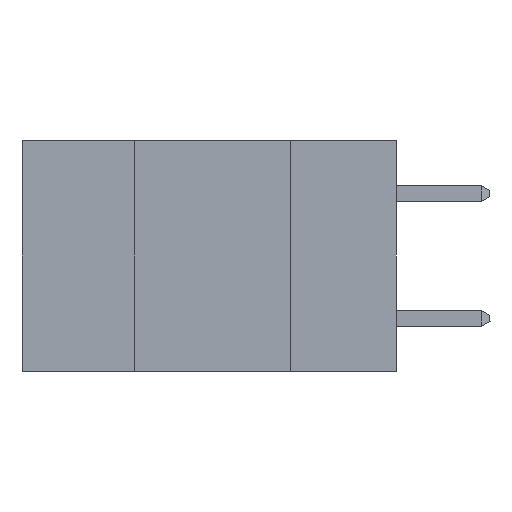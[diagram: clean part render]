
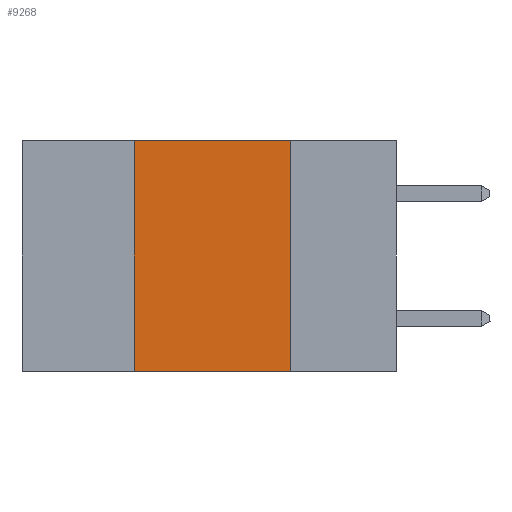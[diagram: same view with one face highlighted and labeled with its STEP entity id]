
A CAD part, left-side view. The second image highlights one B-rep face of the part: STEP entity #9268.
In plain terms, the highlighted planar face has unit normal (-1, 0, 0).
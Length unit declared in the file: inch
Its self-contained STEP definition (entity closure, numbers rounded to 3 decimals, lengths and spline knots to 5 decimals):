
#351 = LINE ( 'NONE', #2457, #1674 ) ;
#396 = VERTEX_POINT ( 'NONE', #8900 ) ;
#916 = VECTOR ( 'NONE', #2219, 39.37008 ) ;
#1001 = EDGE_CURVE ( 'NONE', #5475, #396, #1037, .T. ) ;
#1005 = LINE ( 'NONE', #7188, #9090 ) ;
#1037 = LINE ( 'NONE', #7323, #8994 ) ;
#1189 = PLANE ( 'NONE',  #6844 ) ;
#1674 = VECTOR ( 'NONE', #5648, 39.37008 ) ;
#2209 = CARTESIAN_POINT ( 'NONE',  ( 0., 0.42, -0.37 ) ) ;
#2219 = DIRECTION ( 'NONE',  ( 0., -1., 0. ) ) ;
#2457 = CARTESIAN_POINT ( 'NONE',  ( 0., 0.17, 0. ) ) ;
#2518 = ORIENTED_EDGE ( 'NONE', *, *, #9900, .T. ) ;
#2536 = VERTEX_POINT ( 'NONE', #4464 ) ;
#3486 = DIRECTION ( 'NONE',  ( 1., 0., 0. ) ) ;
#3858 = EDGE_CURVE ( 'NONE', #9818, #2536, #351, .T. ) ;
#4464 = CARTESIAN_POINT ( 'NONE',  ( 0., 0.17, -0.37 ) ) ;
#5098 = LINE ( 'NONE', #8460, #916 ) ;
#5169 = ORIENTED_EDGE ( 'NONE', *, *, #3858, .F. ) ;
#5475 = VERTEX_POINT ( 'NONE', #2209 ) ;
#5648 = DIRECTION ( 'NONE',  ( 0., 0., -1. ) ) ;
#6333 = DIRECTION ( 'NONE',  ( 0., -1., 0. ) ) ;
#6844 = AXIS2_PLACEMENT_3D ( 'NONE', #8904, #3486, #7443 ) ;
#7188 = CARTESIAN_POINT ( 'NONE',  ( 0., 0.6, 0. ) ) ;
#7281 = ORIENTED_EDGE ( 'NONE', *, *, #1001, .F. ) ;
#7323 = CARTESIAN_POINT ( 'NONE',  ( 0., 0.42, 0. ) ) ;
#7443 = DIRECTION ( 'NONE',  ( 0., 0., -1. ) ) ;
#7564 = EDGE_CURVE ( 'NONE', #396, #9818, #1005, .T. ) ;
#7906 = EDGE_LOOP ( 'NONE', ( #5169, #8053, #7281, #2518 ) ) ;
#8053 = ORIENTED_EDGE ( 'NONE', *, *, #7564, .F. ) ;
#8108 = DIRECTION ( 'NONE',  ( 0., 0., 1. ) ) ;
#8431 = CARTESIAN_POINT ( 'NONE',  ( 0., 0.17, 0. ) ) ;
#8460 = CARTESIAN_POINT ( 'NONE',  ( 0., 0.6, -0.37 ) ) ;
#8900 = CARTESIAN_POINT ( 'NONE',  ( 0., 0.42, 0. ) ) ;
#8904 = CARTESIAN_POINT ( 'NONE',  ( 0., 0.6, 0. ) ) ;
#8994 = VECTOR ( 'NONE', #8108, 39.37008 ) ;
#9090 = VECTOR ( 'NONE', #6333, 39.37008 ) ;
#9268 = ADVANCED_FACE ( 'NONE', ( #10006 ), #1189, .F. ) ;
#9818 = VERTEX_POINT ( 'NONE', #8431 ) ;
#9900 = EDGE_CURVE ( 'NONE', #5475, #2536, #5098, .T. ) ;
#10006 = FACE_OUTER_BOUND ( 'NONE', #7906, .T. ) ;
